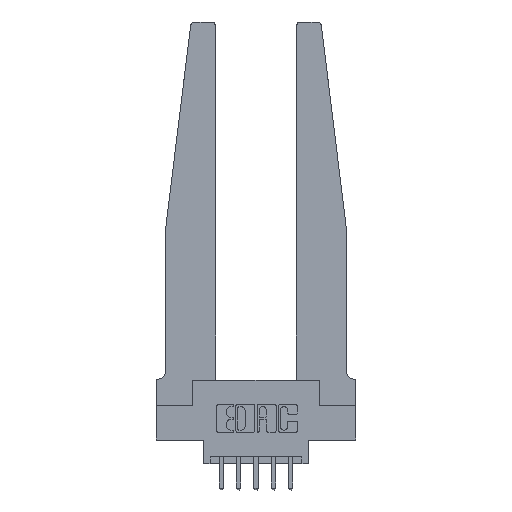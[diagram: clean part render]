
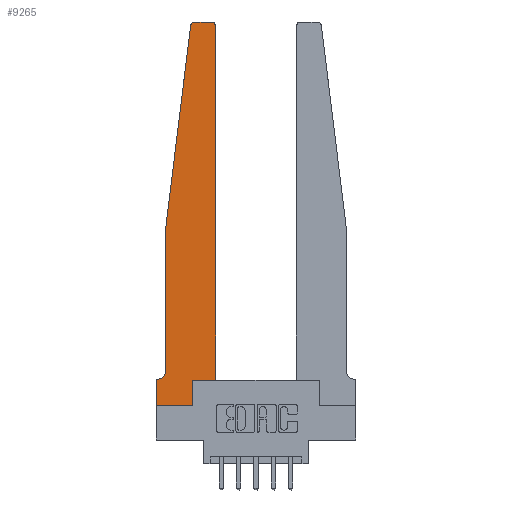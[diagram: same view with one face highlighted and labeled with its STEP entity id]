
A CAD part, top view. The second image highlights one B-rep face of the part: STEP entity #9265.
In plain terms, the highlighted planar face has unit normal (0, 0, 1).
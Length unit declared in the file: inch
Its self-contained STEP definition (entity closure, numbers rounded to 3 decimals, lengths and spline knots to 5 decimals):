
#141 = EDGE_CURVE ( 'NONE', #10182, #2911, #4964, .T. ) ;
#143 = CARTESIAN_POINT ( 'NONE',  ( 0.425, 2.72, 0.37 ) ) ;
#180 = CARTESIAN_POINT ( 'NONE',  ( 0.015, 0.1875, 0.37 ) ) ;
#566 = LINE ( 'NONE', #3635, #10846 ) ;
#630 = ORIENTED_EDGE ( 'NONE', *, *, #8170, .T. ) ;
#681 = VERTEX_POINT ( 'NONE', #969 ) ;
#858 = LINE ( 'NONE', #13424, #2690 ) ;
#950 = VECTOR ( 'NONE', #2989, 39.37008 ) ;
#969 = CARTESIAN_POINT ( 'NONE',  ( 0., 0., 0.37 ) ) ;
#971 = CARTESIAN_POINT ( 'NONE',  ( 0.425, 0.18, 0.37 ) ) ;
#1154 = AXIS2_PLACEMENT_3D ( 'NONE', #1857, #8343, #4285 ) ;
#1164 = ORIENTED_EDGE ( 'NONE', *, *, #2253, .T. ) ;
#1691 = DIRECTION ( 'NONE',  ( 0., 1., 0. ) ) ;
#1857 = CARTESIAN_POINT ( 'NONE',  ( 0.27653, 2.72, 0.37 ) ) ;
#2100 = DIRECTION ( 'NONE',  ( 1., 0., 0. ) ) ;
#2151 = CARTESIAN_POINT ( 'NONE',  ( 0.2605, 0.18, 0.37 ) ) ;
#2200 = CARTESIAN_POINT ( 'NONE',  ( 0.25, 2.75, 0.37 ) ) ;
#2253 = EDGE_CURVE ( 'NONE', #12964, #2324, #3235, .T. ) ;
#2324 = VERTEX_POINT ( 'NONE', #4762 ) ;
#2678 = VERTEX_POINT ( 'NONE', #10873 ) ;
#2690 = VECTOR ( 'NONE', #11403, 39.37008 ) ;
#2799 = AXIS2_PLACEMENT_3D ( 'NONE', #8203, #5110, #4984 ) ;
#2911 = VERTEX_POINT ( 'NONE', #2151 ) ;
#2989 = DIRECTION ( 'NONE',  ( 0., -1., 0. ) ) ;
#3235 = LINE ( 'NONE', #2200, #13272 ) ;
#3285 = CARTESIAN_POINT ( 'NONE',  ( 0.015, 0.2375, 0.37 ) ) ;
#3293 = VERTEX_POINT ( 'NONE', #8212 ) ;
#3392 = VERTEX_POINT ( 'NONE', #180 ) ;
#3506 = FACE_OUTER_BOUND ( 'NONE', #4960, .T. ) ;
#3635 = CARTESIAN_POINT ( 'NONE',  ( 0.425, 0.18, 0.37 ) ) ;
#3684 = LINE ( 'NONE', #4589, #11518 ) ;
#3984 = DIRECTION ( 'NONE',  ( 0., 1., 0. ) ) ;
#4170 = ORIENTED_EDGE ( 'NONE', *, *, #6147, .T. ) ;
#4264 = DIRECTION ( 'NONE',  ( 0., 0., -1. ) ) ;
#4285 = DIRECTION ( 'NONE',  ( 1., 0., 0. ) ) ;
#4288 = CARTESIAN_POINT ( 'NONE',  ( 0.395, 2.75, 0.37 ) ) ;
#4415 = ORIENTED_EDGE ( 'NONE', *, *, #4802, .T. ) ;
#4443 = ORIENTED_EDGE ( 'NONE', *, *, #13547, .T. ) ;
#4502 = VECTOR ( 'NONE', #7923, 39.37008 ) ;
#4589 = CARTESIAN_POINT ( 'NONE',  ( 0., 0., 0.37 ) ) ;
#4676 = VECTOR ( 'NONE', #12289, 39.37008 ) ;
#4762 = CARTESIAN_POINT ( 'NONE',  ( 0.27653, 2.75, 0.37 ) ) ;
#4802 = EDGE_CURVE ( 'NONE', #7455, #6658, #566, .T. ) ;
#4803 = EDGE_CURVE ( 'NONE', #3293, #2678, #9968, .T. ) ;
#4960 = EDGE_LOOP ( 'NONE', ( #1164, #11619, #5239, #9423, #4170, #6271, #4443, #630, #6813, #8077, #4415, #8782 ) ) ;
#4964 = LINE ( 'NONE', #6911, #12749 ) ;
#4984 = DIRECTION ( 'NONE',  ( 1., 0., 0. ) ) ;
#5110 = DIRECTION ( 'NONE',  ( 0., 0., 1. ) ) ;
#5150 = CARTESIAN_POINT ( 'NONE',  ( 0., 0., 0.37 ) ) ;
#5239 = ORIENTED_EDGE ( 'NONE', *, *, #4803, .T. ) ;
#5335 = DIRECTION ( 'NONE',  ( -1., 0., 0. ) ) ;
#5716 = LINE ( 'NONE', #8477, #4502 ) ;
#6147 = EDGE_CURVE ( 'NONE', #9278, #3392, #11647, .T. ) ;
#6271 = ORIENTED_EDGE ( 'NONE', *, *, #8744, .T. ) ;
#6489 = AXIS2_PLACEMENT_3D ( 'NONE', #9845, #12913, #9975 ) ;
#6495 = CIRCLE ( 'NONE', #1154, 0.03 ) ;
#6658 = VERTEX_POINT ( 'NONE', #143 ) ;
#6813 = ORIENTED_EDGE ( 'NONE', *, *, #141, .T. ) ;
#6847 = PLANE ( 'NONE',  #6489 ) ;
#6903 = CARTESIAN_POINT ( 'NONE',  ( 0.065, 1.25, 0.37 ) ) ;
#6911 = CARTESIAN_POINT ( 'NONE',  ( 0.2605, 0.18, 0.37 ) ) ;
#7123 = CARTESIAN_POINT ( 'NONE',  ( 0.425, 0.18, 0.37 ) ) ;
#7424 = EDGE_CURVE ( 'NONE', #6658, #12964, #13429, .T. ) ;
#7455 = VERTEX_POINT ( 'NONE', #7123 ) ;
#7664 = CARTESIAN_POINT ( 'NONE',  ( 0.065, 0.2375, 0.37 ) ) ;
#7695 = EDGE_CURVE ( 'NONE', #2911, #7455, #9411, .T. ) ;
#7908 = DIRECTION ( 'NONE',  ( 1., 0., 0. ) ) ;
#7923 = DIRECTION ( 'NONE',  ( 0., -1., 0. ) ) ;
#8077 = ORIENTED_EDGE ( 'NONE', *, *, #7695, .T. ) ;
#8170 = EDGE_CURVE ( 'NONE', #681, #10182, #3684, .T. ) ;
#8203 = CARTESIAN_POINT ( 'NONE',  ( 0.395, 2.72, 0.37 ) ) ;
#8212 = CARTESIAN_POINT ( 'NONE',  ( 0.24675, 2.72367, 0.37 ) ) ;
#8343 = DIRECTION ( 'NONE',  ( 0., 0., 1. ) ) ;
#8477 = CARTESIAN_POINT ( 'NONE',  ( 0.065, 1.25, 0.37 ) ) ;
#8744 = EDGE_CURVE ( 'NONE', #3392, #9438, #858, .T. ) ;
#8782 = ORIENTED_EDGE ( 'NONE', *, *, #7424, .T. ) ;
#9265 = ADVANCED_FACE ( 'NONE', ( #3506 ), #6847, .T. ) ;
#9278 = VERTEX_POINT ( 'NONE', #7664 ) ;
#9411 = LINE ( 'NONE', #971, #11290 ) ;
#9423 = ORIENTED_EDGE ( 'NONE', *, *, #10712, .T. ) ;
#9438 = VERTEX_POINT ( 'NONE', #13332 ) ;
#9845 = CARTESIAN_POINT ( 'NONE',  ( 0., 0.1875, 0.37 ) ) ;
#9968 = LINE ( 'NONE', #6903, #4676 ) ;
#9975 = DIRECTION ( 'NONE',  ( 1., 0., 0. ) ) ;
#10182 = VERTEX_POINT ( 'NONE', #11273 ) ;
#10712 = EDGE_CURVE ( 'NONE', #2678, #9278, #5716, .T. ) ;
#10846 = VECTOR ( 'NONE', #1691, 39.37008 ) ;
#10873 = CARTESIAN_POINT ( 'NONE',  ( 0.065, 1.25, 0.37 ) ) ;
#11273 = CARTESIAN_POINT ( 'NONE',  ( 0.2605, 0., 0.37 ) ) ;
#11290 = VECTOR ( 'NONE', #2100, 39.37008 ) ;
#11403 = DIRECTION ( 'NONE',  ( -1., 0., 0. ) ) ;
#11518 = VECTOR ( 'NONE', #7908, 39.37008 ) ;
#11619 = ORIENTED_EDGE ( 'NONE', *, *, #11850, .T. ) ;
#11647 = CIRCLE ( 'NONE', #13421, 0.05 ) ;
#11850 = EDGE_CURVE ( 'NONE', #2324, #3293, #6495, .T. ) ;
#12289 = DIRECTION ( 'NONE',  ( -0.122, -0.992, 0. ) ) ;
#12749 = VECTOR ( 'NONE', #3984, 39.37008 ) ;
#12913 = DIRECTION ( 'NONE',  ( 0., 0., 1. ) ) ;
#12964 = VERTEX_POINT ( 'NONE', #4288 ) ;
#12971 = DIRECTION ( 'NONE',  ( -1., 0., 0. ) ) ;
#13272 = VECTOR ( 'NONE', #5335, 39.37008 ) ;
#13332 = CARTESIAN_POINT ( 'NONE',  ( 0., 0.1875, 0.37 ) ) ;
#13421 = AXIS2_PLACEMENT_3D ( 'NONE', #3285, #4264, #12971 ) ;
#13424 = CARTESIAN_POINT ( 'NONE',  ( 0.065, 0.1875, 0.37 ) ) ;
#13429 = CIRCLE ( 'NONE', #2799, 0.03 ) ;
#13453 = LINE ( 'NONE', #5150, #950 ) ;
#13547 = EDGE_CURVE ( 'NONE', #9438, #681, #13453, .T. ) ;
